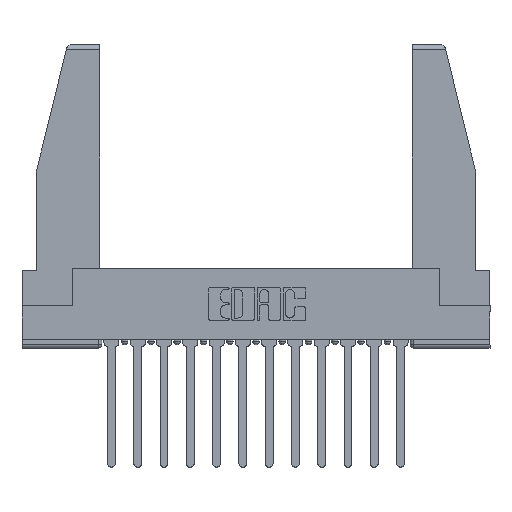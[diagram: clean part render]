
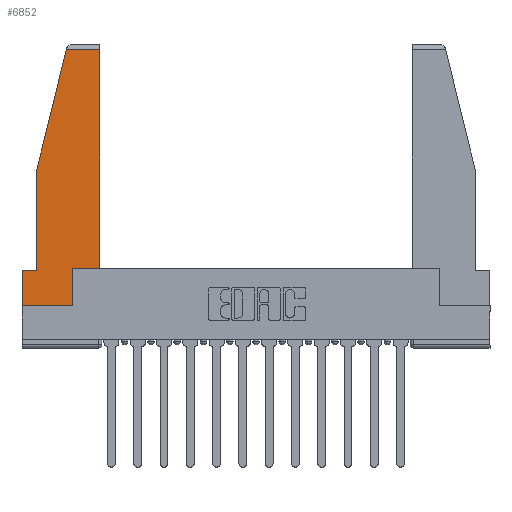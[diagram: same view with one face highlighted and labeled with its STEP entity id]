
A CAD part, top view. The second image highlights one B-rep face of the part: STEP entity #6852.
In plain terms, the highlighted planar face has unit normal (0, 0, 1).
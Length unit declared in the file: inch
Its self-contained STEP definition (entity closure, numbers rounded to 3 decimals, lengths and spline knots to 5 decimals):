
#82 = CARTESIAN_POINT ( 'NONE',  ( 0.461, 0.223, 0. ) ) ;
#389 = DIRECTION ( 'NONE',  ( 0., 1., 0. ) ) ;
#397 = VERTEX_POINT ( 'NONE', #6556 ) ;
#454 = EDGE_CURVE ( 'NONE', #15616, #14572, #1457, .T. ) ;
#770 = DIRECTION ( 'NONE',  ( 1., 0., 0. ) ) ;
#797 = LINE ( 'NONE', #6070, #15785 ) ;
#1253 = ORIENTED_EDGE ( 'NONE', *, *, #10367, .T. ) ;
#1457 = LINE ( 'NONE', #10365, #14036 ) ;
#1514 = ORIENTED_EDGE ( 'NONE', *, *, #8720, .T. ) ;
#1598 = ORIENTED_EDGE ( 'NONE', *, *, #10397, .T. ) ;
#1995 = VERTEX_POINT ( 'NONE', #82 ) ;
#2060 = DIRECTION ( 'NONE',  ( 0., 0., 1. ) ) ;
#2154 = CARTESIAN_POINT ( 'NONE',  ( 0.297, 0., 0. ) ) ;
#2208 = CARTESIAN_POINT ( 'NONE',  ( 0.461, 1.52, 0. ) ) ;
#2291 = CARTESIAN_POINT ( 'NONE',  ( 0., 1.52, 0. ) ) ;
#2863 = LINE ( 'NONE', #7003, #8839 ) ;
#2981 = CARTESIAN_POINT ( 'NONE',  ( 0.086, 0.8, 0. ) ) ;
#3258 = DIRECTION ( 'NONE',  ( 0., -1., 0. ) ) ;
#3419 = PLANE ( 'NONE',  #7188 ) ;
#3677 = VECTOR ( 'NONE', #14890, 39.37008 ) ;
#4252 = VECTOR ( 'NONE', #3258, 39.37008 ) ;
#4421 = ORIENTED_EDGE ( 'NONE', *, *, #14711, .T. ) ;
#4496 = EDGE_CURVE ( 'NONE', #16420, #14297, #797, .T. ) ;
#5164 = CARTESIAN_POINT ( 'NONE',  ( 0.086, 0.21, 0. ) ) ;
#5225 = LINE ( 'NONE', #11612, #11603 ) ;
#5790 = LINE ( 'NONE', #16171, #3677 ) ;
#5987 = DIRECTION ( 'NONE',  ( 1., 0., 0. ) ) ;
#6070 = CARTESIAN_POINT ( 'NONE',  ( 0., 0., 0. ) ) ;
#6113 = LINE ( 'NONE', #2291, #13007 ) ;
#6144 = CARTESIAN_POINT ( 'NONE',  ( 0., 0.21, 0. ) ) ;
#6162 = VECTOR ( 'NONE', #7597, 39.37008 ) ;
#6556 = CARTESIAN_POINT ( 'NONE',  ( 0.297, 0.223, 0. ) ) ;
#6598 = DIRECTION ( 'NONE',  ( 0., -1., 0. ) ) ;
#6852 = ADVANCED_FACE ( 'NONE', ( #13610 ), #3419, .T. ) ;
#6926 = EDGE_CURVE ( 'NONE', #1995, #12723, #5790, .T. ) ;
#7003 = CARTESIAN_POINT ( 'NONE',  ( 0.297, 0., 0. ) ) ;
#7188 = AXIS2_PLACEMENT_3D ( 'NONE', #13698, #2060, #770 ) ;
#7512 = ORIENTED_EDGE ( 'NONE', *, *, #16371, .T. ) ;
#7549 = CARTESIAN_POINT ( 'NONE',  ( 0.297, 0.223, 0. ) ) ;
#7597 = DIRECTION ( 'NONE',  ( -1., 0., 0. ) ) ;
#7672 = CARTESIAN_POINT ( 'NONE',  ( 0.2636, 1.52, 0. ) ) ;
#7762 = LINE ( 'NONE', #6144, #6162 ) ;
#8130 = ORIENTED_EDGE ( 'NONE', *, *, #11495, .T. ) ;
#8572 = LINE ( 'NONE', #7549, #9521 ) ;
#8720 = EDGE_CURVE ( 'NONE', #14297, #397, #2863, .T. ) ;
#8839 = VECTOR ( 'NONE', #389, 39.37008 ) ;
#9390 = ORIENTED_EDGE ( 'NONE', *, *, #6926, .T. ) ;
#9521 = VECTOR ( 'NONE', #13923, 39.37008 ) ;
#9531 = EDGE_LOOP ( 'NONE', ( #9390, #4421, #14675, #8130, #1598, #1253, #13817, #1514, #7512 ) ) ;
#10006 = DIRECTION ( 'NONE',  ( -1., 0., 0. ) ) ;
#10365 = CARTESIAN_POINT ( 'NONE',  ( 0.271, 1.55, 0. ) ) ;
#10367 = EDGE_CURVE ( 'NONE', #11892, #16420, #13537, .T. ) ;
#10397 = EDGE_CURVE ( 'NONE', #16133, #11892, #7762, .T. ) ;
#11495 = EDGE_CURVE ( 'NONE', #14572, #16133, #5225, .T. ) ;
#11603 = VECTOR ( 'NONE', #6598, 39.37008 ) ;
#11612 = CARTESIAN_POINT ( 'NONE',  ( 0.086, 0.8, 0. ) ) ;
#11892 = VERTEX_POINT ( 'NONE', #14065 ) ;
#12723 = VERTEX_POINT ( 'NONE', #2208 ) ;
#12925 = DIRECTION ( 'NONE',  ( -0.239, -0.971, 0. ) ) ;
#13007 = VECTOR ( 'NONE', #10006, 39.37008 ) ;
#13537 = LINE ( 'NONE', #14908, #4252 ) ;
#13610 = FACE_OUTER_BOUND ( 'NONE', #9531, .T. ) ;
#13698 = CARTESIAN_POINT ( 'NONE',  ( 0., 0., 0. ) ) ;
#13817 = ORIENTED_EDGE ( 'NONE', *, *, #4496, .T. ) ;
#13904 = CARTESIAN_POINT ( 'NONE',  ( 0., 0., 0. ) ) ;
#13923 = DIRECTION ( 'NONE',  ( 1., 0., 0. ) ) ;
#14036 = VECTOR ( 'NONE', #12925, 39.37008 ) ;
#14065 = CARTESIAN_POINT ( 'NONE',  ( 0., 0.21, 0. ) ) ;
#14297 = VERTEX_POINT ( 'NONE', #2154 ) ;
#14572 = VERTEX_POINT ( 'NONE', #2981 ) ;
#14675 = ORIENTED_EDGE ( 'NONE', *, *, #454, .T. ) ;
#14711 = EDGE_CURVE ( 'NONE', #12723, #15616, #6113, .T. ) ;
#14890 = DIRECTION ( 'NONE',  ( 0., 1., 0. ) ) ;
#14908 = CARTESIAN_POINT ( 'NONE',  ( 0., 0.21, 0. ) ) ;
#15616 = VERTEX_POINT ( 'NONE', #7672 ) ;
#15785 = VECTOR ( 'NONE', #5987, 39.37008 ) ;
#16133 = VERTEX_POINT ( 'NONE', #5164 ) ;
#16171 = CARTESIAN_POINT ( 'NONE',  ( 0.461, 0.223, 0. ) ) ;
#16371 = EDGE_CURVE ( 'NONE', #397, #1995, #8572, .T. ) ;
#16420 = VERTEX_POINT ( 'NONE', #13904 ) ;
